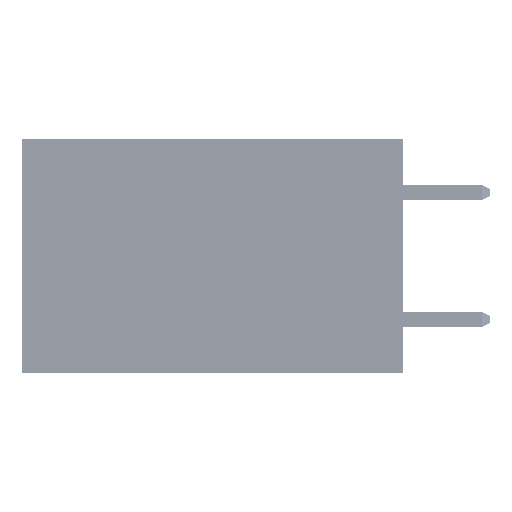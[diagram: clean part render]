
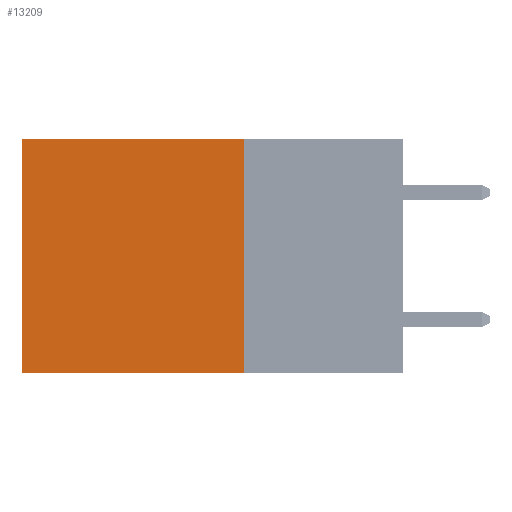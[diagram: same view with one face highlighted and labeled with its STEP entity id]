
A CAD part, left-side view. The second image highlights one B-rep face of the part: STEP entity #13209.
In plain terms, the highlighted planar face has unit normal (-1, 0, 0).
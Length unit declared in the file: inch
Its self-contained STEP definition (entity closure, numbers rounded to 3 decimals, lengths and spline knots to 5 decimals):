
#1379 = CARTESIAN_POINT ( 'NONE',  ( 0.2875, 0.25, -0.37 ) ) ;
#5995 = EDGE_CURVE ( 'NONE', #42450, #37195, #44604, .T. ) ;
#6333 = DIRECTION ( 'NONE',  ( 0., 0., -1. ) ) ;
#7395 = VERTEX_POINT ( 'NONE', #7688 ) ;
#7470 = EDGE_LOOP ( 'NONE', ( #36212, #28216, #45647, #35005 ) ) ;
#7688 = CARTESIAN_POINT ( 'NONE',  ( 0.2875, 0.25, 0. ) ) ;
#9132 = DIRECTION ( 'NONE',  ( 0., 1., 0. ) ) ;
#9927 = PLANE ( 'NONE',  #21565 ) ;
#9928 = VECTOR ( 'NONE', #6333, 39.37008 ) ;
#10166 = DIRECTION ( 'NONE',  ( 1., 0., 0. ) ) ;
#10401 = CARTESIAN_POINT ( 'NONE',  ( 0.2875, 0.25, 0. ) ) ;
#11026 = CARTESIAN_POINT ( 'NONE',  ( 0.2875, 0.6, 0. ) ) ;
#12723 = LINE ( 'NONE', #41790, #14033 ) ;
#13209 = ADVANCED_FACE ( 'NONE', ( #21113 ), #9927, .F. ) ;
#13356 = VECTOR ( 'NONE', #40555, 39.37008 ) ;
#13742 = DIRECTION ( 'NONE',  ( 0., 0., -1. ) ) ;
#14033 = VECTOR ( 'NONE', #9132, 39.37008 ) ;
#15879 = EDGE_CURVE ( 'NONE', #7395, #45124, #12723, .T. ) ;
#18310 = VECTOR ( 'NONE', #29139, 39.37008 ) ;
#20310 = CARTESIAN_POINT ( 'NONE',  ( 0.2875, 0.6, -0.37 ) ) ;
#21113 = FACE_OUTER_BOUND ( 'NONE', #7470, .T. ) ;
#21565 = AXIS2_PLACEMENT_3D ( 'NONE', #10401, #10166, #13742 ) ;
#21736 = LINE ( 'NONE', #31333, #18310 ) ;
#25256 = EDGE_CURVE ( 'NONE', #7395, #42450, #21736, .T. ) ;
#25273 = EDGE_CURVE ( 'NONE', #45124, #37195, #31822, .T. ) ;
#28216 = ORIENTED_EDGE ( 'NONE', *, *, #5995, .F. ) ;
#29139 = DIRECTION ( 'NONE',  ( 0., 0., -1. ) ) ;
#31333 = CARTESIAN_POINT ( 'NONE',  ( 0.2875, 0.25, 0. ) ) ;
#31822 = LINE ( 'NONE', #11026, #9928 ) ;
#35005 = ORIENTED_EDGE ( 'NONE', *, *, #15879, .T. ) ;
#36212 = ORIENTED_EDGE ( 'NONE', *, *, #25273, .T. ) ;
#36751 = CARTESIAN_POINT ( 'NONE',  ( 0.2875, 0.25, -0.37 ) ) ;
#37195 = VERTEX_POINT ( 'NONE', #20310 ) ;
#40555 = DIRECTION ( 'NONE',  ( 0., 1., 0. ) ) ;
#40951 = CARTESIAN_POINT ( 'NONE',  ( 0.2875, 0.6, 0. ) ) ;
#41790 = CARTESIAN_POINT ( 'NONE',  ( 0.2875, 0.25, 0. ) ) ;
#42450 = VERTEX_POINT ( 'NONE', #1379 ) ;
#44604 = LINE ( 'NONE', #36751, #13356 ) ;
#45124 = VERTEX_POINT ( 'NONE', #40951 ) ;
#45647 = ORIENTED_EDGE ( 'NONE', *, *, #25256, .F. ) ;
